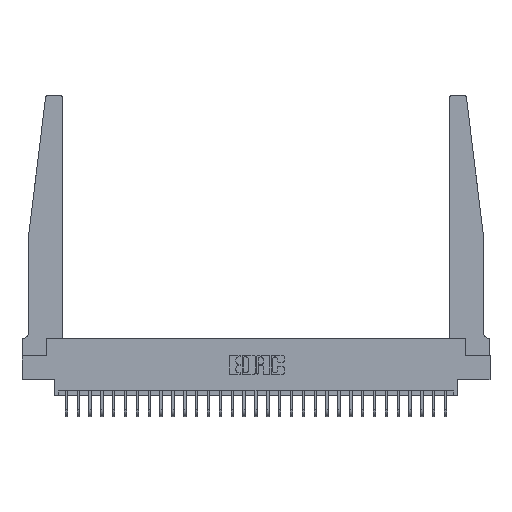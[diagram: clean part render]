
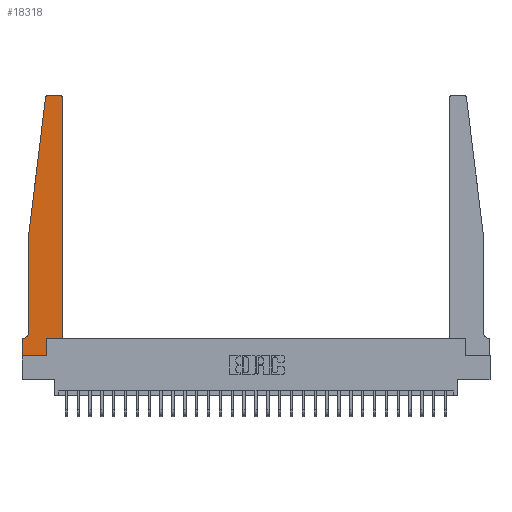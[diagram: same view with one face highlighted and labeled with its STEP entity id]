
A CAD part, top view. The second image highlights one B-rep face of the part: STEP entity #18318.
In plain terms, the highlighted planar face has unit normal (0, 0, 1).
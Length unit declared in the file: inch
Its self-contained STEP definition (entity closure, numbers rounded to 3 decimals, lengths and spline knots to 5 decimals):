
#100 = DIRECTION ( 'NONE',  ( 0., 0., 1. ) ) ;
#441 = VECTOR ( 'NONE', #12967, 39.37008 ) ;
#702 = EDGE_CURVE ( 'NONE', #3715, #16943, #24038, .T. ) ;
#831 = DIRECTION ( 'NONE',  ( -0.122, -0.992, 0. ) ) ;
#1397 = ORIENTED_EDGE ( 'NONE', *, *, #702, .T. ) ;
#1820 = CARTESIAN_POINT ( 'NONE',  ( 0.2605, 0.18, 0.37 ) ) ;
#1854 = ORIENTED_EDGE ( 'NONE', *, *, #28541, .T. ) ;
#1928 = CARTESIAN_POINT ( 'NONE',  ( 0., 0.1875, 0.37 ) ) ;
#2160 = EDGE_LOOP ( 'NONE', ( #10558, #27013, #14412, #2990, #25267, #6105, #8692, #1854, #10680, #1397, #27745, #26491 ) ) ;
#2452 = CARTESIAN_POINT ( 'NONE',  ( 0.395, 2.75, 0.37 ) ) ;
#2568 = VECTOR ( 'NONE', #28520, 39.37008 ) ;
#2990 = ORIENTED_EDGE ( 'NONE', *, *, #6008, .T. ) ;
#3213 = CARTESIAN_POINT ( 'NONE',  ( 0.425, 0.18, 0.37 ) ) ;
#3345 = VECTOR ( 'NONE', #24544, 39.37008 ) ;
#3715 = VERTEX_POINT ( 'NONE', #28732 ) ;
#4045 = CARTESIAN_POINT ( 'NONE',  ( 0.065, 0.2375, 0.37 ) ) ;
#4127 = LINE ( 'NONE', #1820, #7252 ) ;
#4130 = AXIS2_PLACEMENT_3D ( 'NONE', #12643, #16825, #5693 ) ;
#4215 = LINE ( 'NONE', #10690, #441 ) ;
#4501 = VERTEX_POINT ( 'NONE', #18878 ) ;
#5066 = EDGE_CURVE ( 'NONE', #24218, #25767, #4215, .T. ) ;
#5114 = PLANE ( 'NONE',  #12812 ) ;
#5367 = EDGE_CURVE ( 'NONE', #4501, #24218, #24869, .T. ) ;
#5400 = DIRECTION ( 'NONE',  ( 1., 0., 0. ) ) ;
#5693 = DIRECTION ( 'NONE',  ( -1., 0., 0. ) ) ;
#6008 = EDGE_CURVE ( 'NONE', #27678, #17295, #7582, .T. ) ;
#6053 = DIRECTION ( 'NONE',  ( 1., 0., 0. ) ) ;
#6096 = CARTESIAN_POINT ( 'NONE',  ( 0.425, 0.18, 0.37 ) ) ;
#6105 = ORIENTED_EDGE ( 'NONE', *, *, #5367, .T. ) ;
#6358 = DIRECTION ( 'NONE',  ( 1., 0., 0. ) ) ;
#6936 = FACE_OUTER_BOUND ( 'NONE', #2160, .T. ) ;
#7252 = VECTOR ( 'NONE', #29351, 39.37008 ) ;
#7582 = LINE ( 'NONE', #16733, #8733 ) ;
#7768 = AXIS2_PLACEMENT_3D ( 'NONE', #25415, #13180, #6358 ) ;
#7813 = LINE ( 'NONE', #15036, #23872 ) ;
#8692 = ORIENTED_EDGE ( 'NONE', *, *, #5066, .T. ) ;
#8733 = VECTOR ( 'NONE', #12395, 39.37008 ) ;
#9337 = CARTESIAN_POINT ( 'NONE',  ( 0.425, 0.18, 0.37 ) ) ;
#10558 = ORIENTED_EDGE ( 'NONE', *, *, #16573, .T. ) ;
#10651 = CARTESIAN_POINT ( 'NONE',  ( 0.065, 0.1875, 0.37 ) ) ;
#10680 = ORIENTED_EDGE ( 'NONE', *, *, #22652, .T. ) ;
#10690 = CARTESIAN_POINT ( 'NONE',  ( 0., 0., 0.37 ) ) ;
#10761 = VECTOR ( 'NONE', #29640, 39.37008 ) ;
#10770 = AXIS2_PLACEMENT_3D ( 'NONE', #28888, #29042, #6053 ) ;
#11498 = LINE ( 'NONE', #15836, #10761 ) ;
#11711 = CARTESIAN_POINT ( 'NONE',  ( 0.24675, 2.72367, 0.37 ) ) ;
#12395 = DIRECTION ( 'NONE',  ( 0., -1., 0. ) ) ;
#12643 = CARTESIAN_POINT ( 'NONE',  ( 0.015, 0.2375, 0.37 ) ) ;
#12696 = CARTESIAN_POINT ( 'NONE',  ( 0., 0., 0.37 ) ) ;
#12812 = AXIS2_PLACEMENT_3D ( 'NONE', #23068, #100, #5400 ) ;
#12967 = DIRECTION ( 'NONE',  ( 0., -1., 0. ) ) ;
#13180 = DIRECTION ( 'NONE',  ( 0., 0., 1. ) ) ;
#14206 = CARTESIAN_POINT ( 'NONE',  ( 0.27653, 2.75, 0.37 ) ) ;
#14412 = ORIENTED_EDGE ( 'NONE', *, *, #18335, .T. ) ;
#15036 = CARTESIAN_POINT ( 'NONE',  ( 0.065, 1.25, 0.37 ) ) ;
#15418 = VECTOR ( 'NONE', #24238, 39.37008 ) ;
#15432 = CIRCLE ( 'NONE', #7768, 0.03 ) ;
#15836 = CARTESIAN_POINT ( 'NONE',  ( 0., 0., 0.37 ) ) ;
#16545 = VERTEX_POINT ( 'NONE', #28384 ) ;
#16573 = EDGE_CURVE ( 'NONE', #23851, #22831, #26555, .T. ) ;
#16733 = CARTESIAN_POINT ( 'NONE',  ( 0.065, 1.25, 0.37 ) ) ;
#16825 = DIRECTION ( 'NONE',  ( 0., 0., -1. ) ) ;
#16943 = VERTEX_POINT ( 'NONE', #9337 ) ;
#17176 = VERTEX_POINT ( 'NONE', #19248 ) ;
#17295 = VERTEX_POINT ( 'NONE', #4045 ) ;
#17561 = CIRCLE ( 'NONE', #4130, 0.05 ) ;
#18074 = CARTESIAN_POINT ( 'NONE',  ( 0.065, 1.25, 0.37 ) ) ;
#18318 = ADVANCED_FACE ( 'NONE', ( #6936 ), #5114, .T. ) ;
#18328 = EDGE_CURVE ( 'NONE', #17295, #4501, #17561, .T. ) ;
#18335 = EDGE_CURVE ( 'NONE', #29526, #27678, #7813, .T. ) ;
#18878 = CARTESIAN_POINT ( 'NONE',  ( 0.015, 0.1875, 0.37 ) ) ;
#19248 = CARTESIAN_POINT ( 'NONE',  ( 0.2605, 0., 0.37 ) ) ;
#22652 = EDGE_CURVE ( 'NONE', #17176, #3715, #4127, .T. ) ;
#22684 = EDGE_CURVE ( 'NONE', #16545, #23851, #15432, .T. ) ;
#22831 = VERTEX_POINT ( 'NONE', #14206 ) ;
#23068 = CARTESIAN_POINT ( 'NONE',  ( 0., 0.1875, 0.37 ) ) ;
#23851 = VERTEX_POINT ( 'NONE', #2452 ) ;
#23872 = VECTOR ( 'NONE', #831, 39.37008 ) ;
#24038 = LINE ( 'NONE', #3213, #27274 ) ;
#24218 = VERTEX_POINT ( 'NONE', #1928 ) ;
#24238 = DIRECTION ( 'NONE',  ( -1., 0., 0. ) ) ;
#24544 = DIRECTION ( 'NONE',  ( 0., 1., 0. ) ) ;
#24869 = LINE ( 'NONE', #10651, #15418 ) ;
#25267 = ORIENTED_EDGE ( 'NONE', *, *, #18328, .T. ) ;
#25415 = CARTESIAN_POINT ( 'NONE',  ( 0.395, 2.72, 0.37 ) ) ;
#25767 = VERTEX_POINT ( 'NONE', #12696 ) ;
#26349 = DIRECTION ( 'NONE',  ( 1., 0., 0. ) ) ;
#26491 = ORIENTED_EDGE ( 'NONE', *, *, #22684, .T. ) ;
#26555 = LINE ( 'NONE', #28676, #2568 ) ;
#26827 = LINE ( 'NONE', #6096, #3345 ) ;
#27013 = ORIENTED_EDGE ( 'NONE', *, *, #27049, .T. ) ;
#27049 = EDGE_CURVE ( 'NONE', #22831, #29526, #27673, .T. ) ;
#27274 = VECTOR ( 'NONE', #26349, 39.37008 ) ;
#27673 = CIRCLE ( 'NONE', #10770, 0.03 ) ;
#27678 = VERTEX_POINT ( 'NONE', #18074 ) ;
#27745 = ORIENTED_EDGE ( 'NONE', *, *, #28102, .T. ) ;
#28102 = EDGE_CURVE ( 'NONE', #16943, #16545, #26827, .T. ) ;
#28384 = CARTESIAN_POINT ( 'NONE',  ( 0.425, 2.72, 0.37 ) ) ;
#28520 = DIRECTION ( 'NONE',  ( -1., 0., 0. ) ) ;
#28541 = EDGE_CURVE ( 'NONE', #25767, #17176, #11498, .T. ) ;
#28676 = CARTESIAN_POINT ( 'NONE',  ( 0.25, 2.75, 0.37 ) ) ;
#28732 = CARTESIAN_POINT ( 'NONE',  ( 0.2605, 0.18, 0.37 ) ) ;
#28888 = CARTESIAN_POINT ( 'NONE',  ( 0.27653, 2.72, 0.37 ) ) ;
#29042 = DIRECTION ( 'NONE',  ( 0., 0., 1. ) ) ;
#29351 = DIRECTION ( 'NONE',  ( 0., 1., 0. ) ) ;
#29526 = VERTEX_POINT ( 'NONE', #11711 ) ;
#29640 = DIRECTION ( 'NONE',  ( 1., 0., 0. ) ) ;
